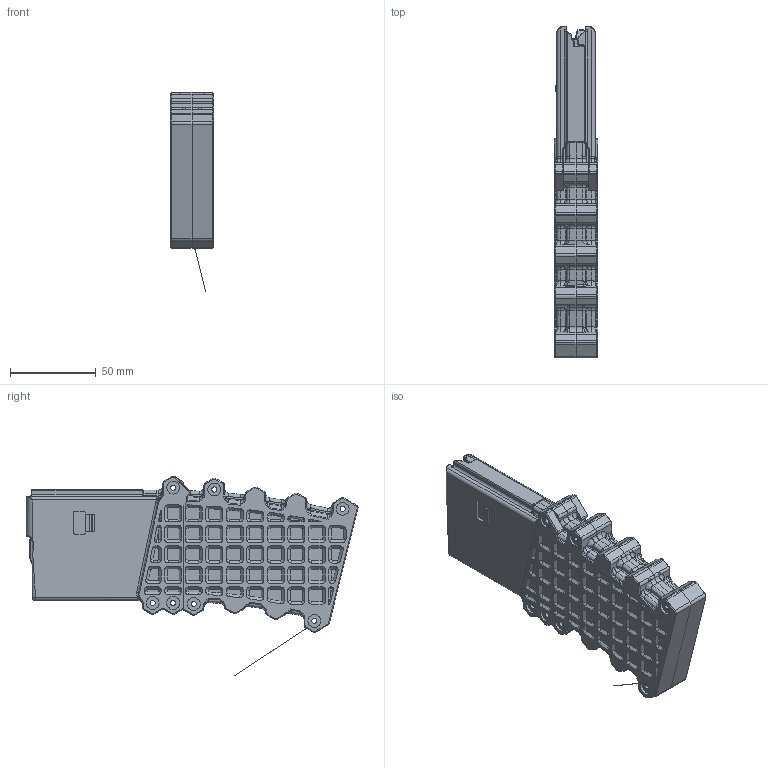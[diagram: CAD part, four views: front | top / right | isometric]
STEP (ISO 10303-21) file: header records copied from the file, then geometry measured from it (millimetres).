
FILE_DESCRIPTION (( 'STEP AP214' ), '1' );
FILE_NAME ('Waffle Magazine.STEP', '2021-05-01T22:58:08', ( '' ), ( '' ), 'SwSTEP 2.0', 'SolidWorks 2020', '' );
FILE_SCHEMA (( 'AUTOMOTIVE_DESIGN' ));
Length unit declared in the file: millimetre
Products named in the file (5): Mag Body Bottom Right; Mag Body Bottom Left; Mag Follower; Waffle Magazine; Mag Body Top
Assembly tree (4 placements, depth 2):
  Waffle Magazine
    Mag Body Top
    Mag Body Bottom Left
    Mag Body Bottom Right
    Mag Follower
Bounding box: 25.5 x 194 x 116.49 mm (x, y, z)
Volume: 117879.3 mm3; surface area: 82430.9 mm2
Topology: 4 solids, 5 shells, 3095 faces, 7949 edges, 4872 vertices
Faces by surface type: plane 973, cylinder 803, bspline 639, cone 478, torus 172, sphere 30
Entity records: 117517 total; most frequent: CARTESIAN_POINT 47237, ORIENTED_EDGE 15650, DIRECTION 13498, EDGE_CURVE 7825, AXIS2_PLACEMENT_3D 4966, VERTEX_POINT 4864, VECTOR 3566, LINE 3566
